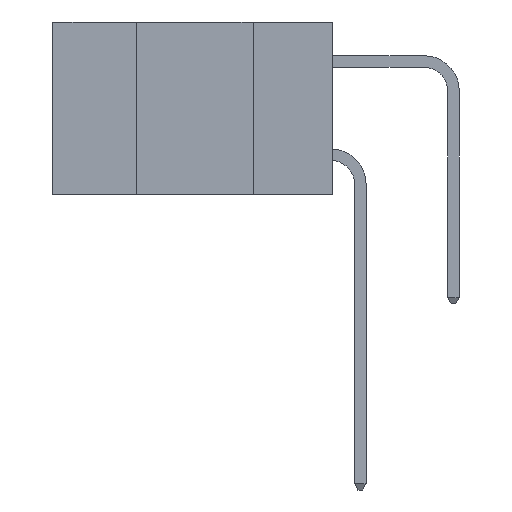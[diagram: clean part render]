
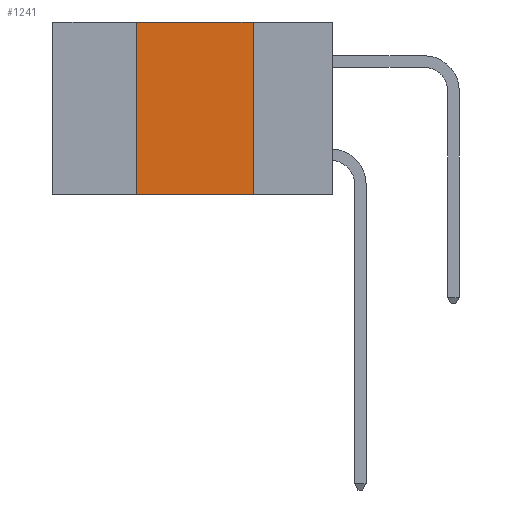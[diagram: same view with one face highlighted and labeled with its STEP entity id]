
A CAD part, left-side view. The second image highlights one B-rep face of the part: STEP entity #1241.
In plain terms, the highlighted planar face has unit normal (-1, 0, 0).
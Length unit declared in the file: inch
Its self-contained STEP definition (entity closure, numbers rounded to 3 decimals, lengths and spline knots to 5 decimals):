
#284 = CARTESIAN_POINT ( 'NONE',  ( 0., 0.6, 0. ) ) ;
#536 = PLANE ( 'NONE',  #8276 ) ;
#596 = DIRECTION ( 'NONE',  ( 0., -1., 0. ) ) ;
#640 = EDGE_LOOP ( 'NONE', ( #8220, #9732, #5796, #4598 ) ) ;
#671 = CARTESIAN_POINT ( 'NONE',  ( 0., 0.17, -0.37 ) ) ;
#725 = CARTESIAN_POINT ( 'NONE',  ( 0., 0.17, 0. ) ) ;
#1079 = LINE ( 'NONE', #10131, #5323 ) ;
#1241 = ADVANCED_FACE ( 'NONE', ( #8745 ), #536, .F. ) ;
#1603 = VERTEX_POINT ( 'NONE', #671 ) ;
#1835 = EDGE_CURVE ( 'NONE', #9694, #7450, #8009, .T. ) ;
#2432 = VECTOR ( 'NONE', #7620, 39.37008 ) ;
#3044 = CARTESIAN_POINT ( 'NONE',  ( 0., 0.6, 0. ) ) ;
#3466 = CARTESIAN_POINT ( 'NONE',  ( 0., 0.42, 0. ) ) ;
#3644 = DIRECTION ( 'NONE',  ( 0., 0., 1. ) ) ;
#3960 = CARTESIAN_POINT ( 'NONE',  ( 0., 0.42, -0.37 ) ) ;
#4598 = ORIENTED_EDGE ( 'NONE', *, *, #5277, .T. ) ;
#5277 = EDGE_CURVE ( 'NONE', #9694, #1603, #1079, .T. ) ;
#5323 = VECTOR ( 'NONE', #596, 39.37008 ) ;
#5676 = CARTESIAN_POINT ( 'NONE',  ( 0., 0.17, -0.37 ) ) ;
#5796 = ORIENTED_EDGE ( 'NONE', *, *, #1835, .F. ) ;
#5806 = VECTOR ( 'NONE', #3644, 39.37008 ) ;
#6435 = DIRECTION ( 'NONE',  ( 0., 0., -1. ) ) ;
#6459 = VERTEX_POINT ( 'NONE', #725 ) ;
#6883 = EDGE_CURVE ( 'NONE', #7450, #6459, #8538, .T. ) ;
#7450 = VERTEX_POINT ( 'NONE', #3466 ) ;
#7620 = DIRECTION ( 'NONE',  ( 0., -1., 0. ) ) ;
#7867 = EDGE_CURVE ( 'NONE', #6459, #1603, #8867, .T. ) ;
#8009 = LINE ( 'NONE', #3960, #5806 ) ;
#8220 = ORIENTED_EDGE ( 'NONE', *, *, #7867, .F. ) ;
#8276 = AXIS2_PLACEMENT_3D ( 'NONE', #284, #10405, #10373 ) ;
#8538 = LINE ( 'NONE', #3044, #2432 ) ;
#8745 = FACE_OUTER_BOUND ( 'NONE', #640, .T. ) ;
#8867 = LINE ( 'NONE', #5676, #9087 ) ;
#9087 = VECTOR ( 'NONE', #6435, 39.37008 ) ;
#9694 = VERTEX_POINT ( 'NONE', #9850 ) ;
#9732 = ORIENTED_EDGE ( 'NONE', *, *, #6883, .F. ) ;
#9850 = CARTESIAN_POINT ( 'NONE',  ( 0., 0.42, -0.37 ) ) ;
#10131 = CARTESIAN_POINT ( 'NONE',  ( 0., 0.6, -0.37 ) ) ;
#10373 = DIRECTION ( 'NONE',  ( 0., 0., -1. ) ) ;
#10405 = DIRECTION ( 'NONE',  ( 1., 0., 0. ) ) ;
